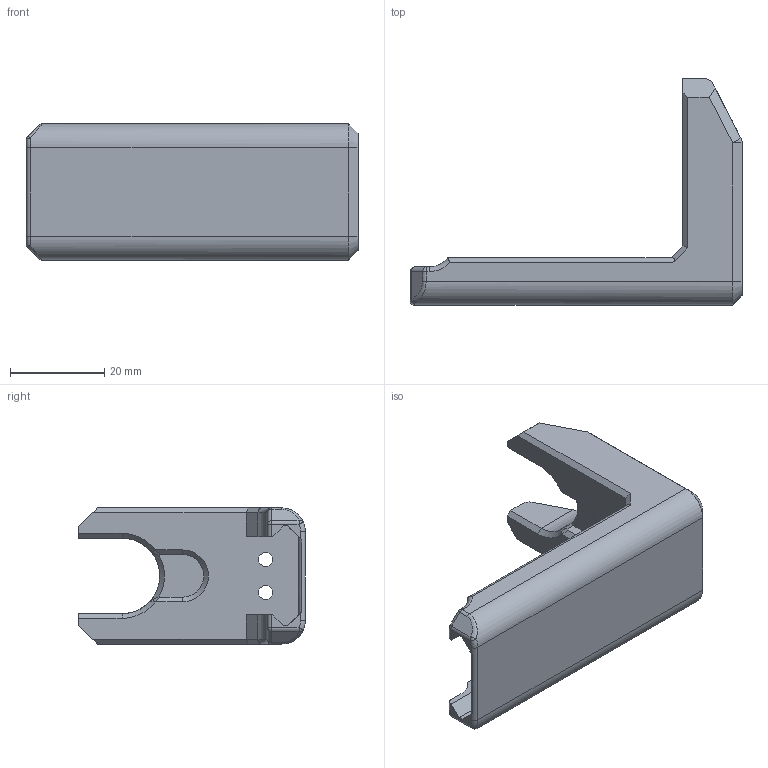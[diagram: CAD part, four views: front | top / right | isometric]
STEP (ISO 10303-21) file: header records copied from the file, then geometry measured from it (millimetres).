
FILE_DESCRIPTION(/* description */ (''),/* implementation_level */ '2;1');
FILE_NAME(/* name */ 'G1926 Standoff.step',/* time_stamp */ '2022-07-20T09:40:55-06:00',/* author */ (''),/* organization */ (''),/* preprocessor_version */ 'ST-DEVELOPER v19',/* originating_system */ 'Autodesk Translation Framework v11.7.0.108',/* authorisation */ '');
FILE_SCHEMA (('AUTOMOTIVE_DESIGN { 1 0 10303 214 3 1 1 }'));
Length unit declared in the file: millimetre
Products named in the file (1): G19/26
Bounding box: 70.38 x 48.03 x 28.86 mm (x, y, z)
Volume: 19284.2 mm3; surface area: 10181.9 mm2
Topology: 1 solids, 1 shells, 654 faces, 1722 edges, 1138 vertices
Faces by surface type: bspline 451, plane 140, cylinder 45, cone 8, sphere 6, torus 4
Full cylindrical faces by diameter (mm): 3 x2, 5.5 x2
Entity records: 21812 total; most frequent: CARTESIAN_POINT 9588, ORIENTED_EDGE 3440, EDGE_CURVE 1720, DIRECTION 1312, VERTEX_POINT 1138, EDGE_LOOP 728, LINE 684, VECTOR 684
